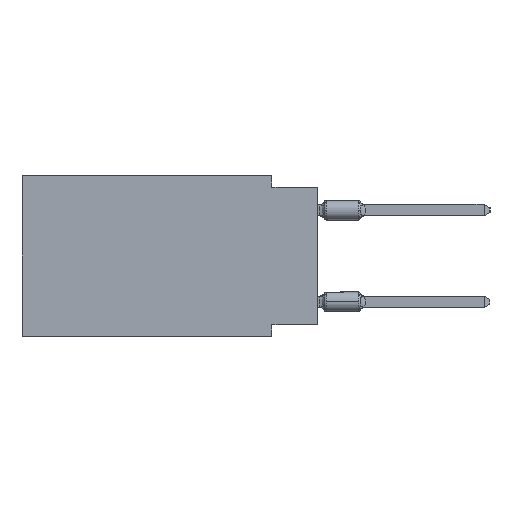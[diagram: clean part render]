
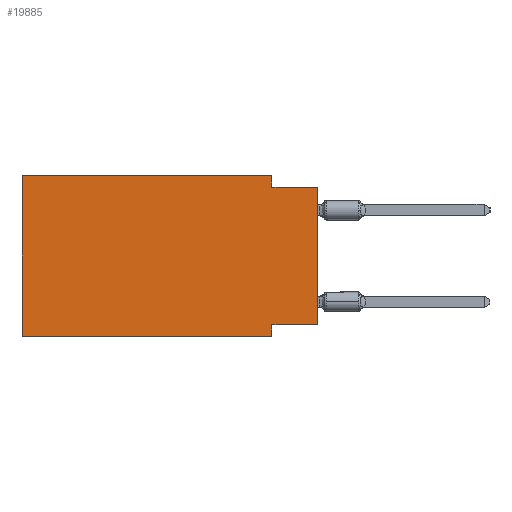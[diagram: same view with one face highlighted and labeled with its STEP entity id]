
A CAD part, left-side view. The second image highlights one B-rep face of the part: STEP entity #19885.
In plain terms, the highlighted planar face has unit normal (-1, 0, 0).
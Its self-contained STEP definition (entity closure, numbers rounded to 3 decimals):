
#52 = CARTESIAN_POINT ( 'NONE',  ( 0., 16.383, 0. ) ) ;
#128 = CARTESIAN_POINT ( 'NONE',  ( 0., 2.54, -0.635 ) ) ;
#2483 = ORIENTED_EDGE ( 'NONE', *, *, #5803, .F. ) ;
#3521 = DIRECTION ( 'NONE',  ( 0., 0., -1. ) ) ;
#5601 = VERTEX_POINT ( 'NONE', #7554 ) ;
#5782 = DIRECTION ( 'NONE',  ( 0., 0., -1. ) ) ;
#5803 = EDGE_CURVE ( 'NONE', #8412, #23947, #8096, .T. ) ;
#6233 = DIRECTION ( 'NONE',  ( 0., 0., 1. ) ) ;
#7554 = CARTESIAN_POINT ( 'NONE',  ( 0., 0., -8.255 ) ) ;
#8096 = LINE ( 'NONE', #52, #44926 ) ;
#8412 = VERTEX_POINT ( 'NONE', #32108 ) ;
#9242 = ORIENTED_EDGE ( 'NONE', *, *, #42366, .F. ) ;
#9493 = ORIENTED_EDGE ( 'NONE', *, *, #9926, .F. ) ;
#9926 = EDGE_CURVE ( 'NONE', #5601, #37953, #21019, .T. ) ;
#10802 = VERTEX_POINT ( 'NONE', #34431 ) ;
#11739 = VECTOR ( 'NONE', #22857, 1000. ) ;
#12776 = LINE ( 'NONE', #29132, #33018 ) ;
#13169 = FACE_OUTER_BOUND ( 'NONE', #21929, .T. ) ;
#13847 = ORIENTED_EDGE ( 'NONE', *, *, #26135, .F. ) ;
#14211 = VERTEX_POINT ( 'NONE', #14477 ) ;
#14477 = CARTESIAN_POINT ( 'NONE',  ( 0., 2.54, -8.89 ) ) ;
#16402 = CARTESIAN_POINT ( 'NONE',  ( 0., 16.383, 0. ) ) ;
#16606 = ORIENTED_EDGE ( 'NONE', *, *, #34036, .F. ) ;
#16819 = LINE ( 'NONE', #37823, #30341 ) ;
#16881 = CARTESIAN_POINT ( 'NONE',  ( 0., 0., -8.255 ) ) ;
#17676 = VERTEX_POINT ( 'NONE', #18934 ) ;
#17853 = DIRECTION ( 'NONE',  ( 1., 0., 0. ) ) ;
#18257 = LINE ( 'NONE', #30448, #29215 ) ;
#18934 = CARTESIAN_POINT ( 'NONE',  ( 0., 0., -0.635 ) ) ;
#19814 = VERTEX_POINT ( 'NONE', #128 ) ;
#19885 = ADVANCED_FACE ( 'NONE', ( #13169 ), #33922, .F. ) ;
#21019 = LINE ( 'NONE', #16881, #32799 ) ;
#21929 = EDGE_LOOP ( 'NONE', ( #50732, #16606, #9242, #52006, #2483, #28020, #13847, #9493 ) ) ;
#22857 = DIRECTION ( 'NONE',  ( 0., -1., 0. ) ) ;
#23947 = VERTEX_POINT ( 'NONE', #53425 ) ;
#24370 = DIRECTION ( 'NONE',  ( 0., 1., 0. ) ) ;
#24434 = DIRECTION ( 'NONE',  ( 0., -1., 0. ) ) ;
#26135 = EDGE_CURVE ( 'NONE', #37953, #14211, #18257, .T. ) ;
#27830 = LINE ( 'NONE', #52402, #11739 ) ;
#28020 = ORIENTED_EDGE ( 'NONE', *, *, #50269, .T. ) ;
#29132 = CARTESIAN_POINT ( 'NONE',  ( 0., 0., -0.635 ) ) ;
#29215 = VECTOR ( 'NONE', #5782, 1000. ) ;
#30071 = AXIS2_PLACEMENT_3D ( 'NONE', #42221, #17853, #38880 ) ;
#30341 = VECTOR ( 'NONE', #3521, 1000. ) ;
#30448 = CARTESIAN_POINT ( 'NONE',  ( 0., 2.54, -8.89 ) ) ;
#30885 = CARTESIAN_POINT ( 'NONE',  ( 0., 0., 0. ) ) ;
#32108 = CARTESIAN_POINT ( 'NONE',  ( 0., 16.383, -8.89 ) ) ;
#32799 = VECTOR ( 'NONE', #24370, 1000. ) ;
#33018 = VECTOR ( 'NONE', #24434, 1000. ) ;
#33841 = DIRECTION ( 'NONE',  ( 0., 0., 1. ) ) ;
#33922 = PLANE ( 'NONE',  #30071 ) ;
#34036 = EDGE_CURVE ( 'NONE', #19814, #17676, #12776, .T. ) ;
#34045 = VECTOR ( 'NONE', #6233, 1000. ) ;
#34155 = EDGE_CURVE ( 'NONE', #23947, #10802, #41569, .T. ) ;
#34431 = CARTESIAN_POINT ( 'NONE',  ( 0., 2.54, 0. ) ) ;
#37384 = CARTESIAN_POINT ( 'NONE',  ( 0., 2.54, -8.255 ) ) ;
#37823 = CARTESIAN_POINT ( 'NONE',  ( 0., 2.54, 0. ) ) ;
#37953 = VERTEX_POINT ( 'NONE', #37384 ) ;
#38299 = VECTOR ( 'NONE', #50115, 1000. ) ;
#38880 = DIRECTION ( 'NONE',  ( 0., 0., -1. ) ) ;
#41569 = LINE ( 'NONE', #16402, #38299 ) ;
#42221 = CARTESIAN_POINT ( 'NONE',  ( 0., 16.383, 0. ) ) ;
#42366 = EDGE_CURVE ( 'NONE', #10802, #19814, #16819, .T. ) ;
#44299 = EDGE_CURVE ( 'NONE', #5601, #17676, #52149, .T. ) ;
#44926 = VECTOR ( 'NONE', #33841, 1000. ) ;
#50115 = DIRECTION ( 'NONE',  ( 0., -1., 0. ) ) ;
#50269 = EDGE_CURVE ( 'NONE', #8412, #14211, #27830, .T. ) ;
#50732 = ORIENTED_EDGE ( 'NONE', *, *, #44299, .T. ) ;
#52006 = ORIENTED_EDGE ( 'NONE', *, *, #34155, .F. ) ;
#52149 = LINE ( 'NONE', #30885, #34045 ) ;
#52402 = CARTESIAN_POINT ( 'NONE',  ( 0., 16.383, -8.89 ) ) ;
#53425 = CARTESIAN_POINT ( 'NONE',  ( 0., 16.383, 0. ) ) ;
